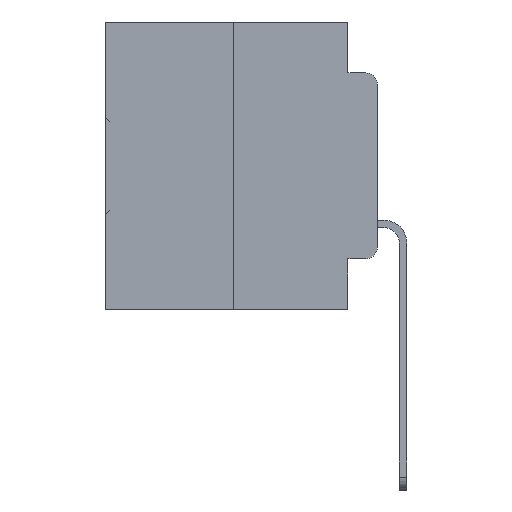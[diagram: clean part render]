
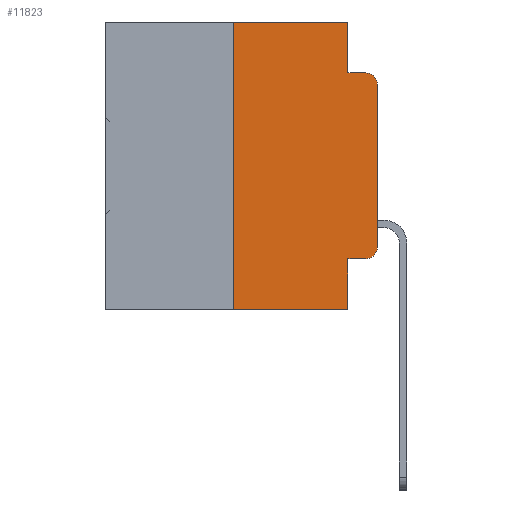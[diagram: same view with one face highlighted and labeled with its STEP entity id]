
A CAD part, left-side view. The second image highlights one B-rep face of the part: STEP entity #11823.
In plain terms, the highlighted planar face has unit normal (-1, 0, 0).
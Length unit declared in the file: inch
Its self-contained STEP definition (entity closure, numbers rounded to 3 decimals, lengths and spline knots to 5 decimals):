
#472 = CIRCLE ( 'NONE', #4220, 0.02 ) ;
#721 = CARTESIAN_POINT ( 'NONE',  ( 0., 0.473, -0.5 ) ) ;
#1151 = VECTOR ( 'NONE', #5588, 39.37008 ) ;
#1259 = ORIENTED_EDGE ( 'NONE', *, *, #29173, .F. ) ;
#1295 = EDGE_CURVE ( 'NONE', #19458, #22076, #29557, .T. ) ;
#1389 = ORIENTED_EDGE ( 'NONE', *, *, #27948, .F. ) ;
#1574 = DIRECTION ( 'NONE',  ( -1., 0., 0. ) ) ;
#1918 = ORIENTED_EDGE ( 'NONE', *, *, #8232, .T. ) ;
#2034 = ORIENTED_EDGE ( 'NONE', *, *, #1295, .T. ) ;
#2562 = LINE ( 'NONE', #23616, #16361 ) ;
#3032 = CARTESIAN_POINT ( 'NONE',  ( 0., 0.02, -0.1085 ) ) ;
#3521 = ORIENTED_EDGE ( 'NONE', *, *, #4174, .F. ) ;
#3566 = ORIENTED_EDGE ( 'NONE', *, *, #13901, .T. ) ;
#3948 = ORIENTED_EDGE ( 'NONE', *, *, #20472, .F. ) ;
#4174 = EDGE_CURVE ( 'NONE', #14409, #23871, #2562, .T. ) ;
#4220 = AXIS2_PLACEMENT_3D ( 'NONE', #18085, #1574, #20760 ) ;
#4297 = DIRECTION ( 'NONE',  ( 0., -1., 0. ) ) ;
#4519 = DIRECTION ( 'NONE',  ( 0., 0., 1. ) ) ;
#4580 = DIRECTION ( 'NONE',  ( 0., 0., -1. ) ) ;
#4784 = ORIENTED_EDGE ( 'NONE', *, *, #31657, .F. ) ;
#4877 = VECTOR ( 'NONE', #19942, 39.37008 ) ;
#5535 = ORIENTED_EDGE ( 'NONE', *, *, #14051, .T. ) ;
#5543 = CARTESIAN_POINT ( 'NONE',  ( 0., 0.051, -0.4115 ) ) ;
#5588 = DIRECTION ( 'NONE',  ( 0., 0., 1. ) ) ;
#5864 = DIRECTION ( 'NONE',  ( 0., 0., -1. ) ) ;
#6602 = DIRECTION ( 'NONE',  ( 0., 0., -1. ) ) ;
#7320 = DIRECTION ( 'NONE',  ( 0., 0., -1. ) ) ;
#8232 = EDGE_CURVE ( 'NONE', #28166, #24749, #30125, .T. ) ;
#8247 = CARTESIAN_POINT ( 'NONE',  ( 0., 0., -0.3915 ) ) ;
#8298 = CARTESIAN_POINT ( 'NONE',  ( 0., 0., -0.1085 ) ) ;
#8684 = CARTESIAN_POINT ( 'NONE',  ( 0., 0.051, 0. ) ) ;
#9003 = ORIENTED_EDGE ( 'NONE', *, *, #16883, .T. ) ;
#9550 = CARTESIAN_POINT ( 'NONE',  ( 0., 0.473, 0. ) ) ;
#11013 = AXIS2_PLACEMENT_3D ( 'NONE', #3032, #22141, #5864 ) ;
#11559 = CIRCLE ( 'NONE', #11013, 0.02 ) ;
#11646 = CARTESIAN_POINT ( 'NONE',  ( 0., 0.051, -0.5 ) ) ;
#11823 = ADVANCED_FACE ( 'NONE', ( #32432 ), #33493, .F. ) ;
#13744 = LINE ( 'NONE', #17960, #28013 ) ;
#13901 = EDGE_CURVE ( 'NONE', #33383, #34877, #26547, .T. ) ;
#14051 = EDGE_CURVE ( 'NONE', #22076, #28166, #472, .T. ) ;
#14409 = VERTEX_POINT ( 'NONE', #8684 ) ;
#15096 = VERTEX_POINT ( 'NONE', #19532 ) ;
#15580 = CARTESIAN_POINT ( 'NONE',  ( 0., 0.25, 0. ) ) ;
#15777 = CARTESIAN_POINT ( 'NONE',  ( 0., 0.051, -0.4115 ) ) ;
#16361 = VECTOR ( 'NONE', #4580, 39.37008 ) ;
#16883 = EDGE_CURVE ( 'NONE', #24749, #22180, #11559, .T. ) ;
#17960 = CARTESIAN_POINT ( 'NONE',  ( 0., 0.051, -0.0885 ) ) ;
#18085 = CARTESIAN_POINT ( 'NONE',  ( 0., 0.02, -0.3915 ) ) ;
#19458 = VERTEX_POINT ( 'NONE', #5543 ) ;
#19532 = CARTESIAN_POINT ( 'NONE',  ( 0., 0.25, 0. ) ) ;
#19942 = DIRECTION ( 'NONE',  ( 0., -1., 0. ) ) ;
#20000 = EDGE_LOOP ( 'NONE', ( #1918, #9003, #4784, #3521, #1389, #1259, #3566, #3948, #2034, #5535 ) ) ;
#20144 = CARTESIAN_POINT ( 'NONE',  ( 0., 0.473, 0. ) ) ;
#20472 = EDGE_CURVE ( 'NONE', #19458, #34877, #27426, .T. ) ;
#20760 = DIRECTION ( 'NONE',  ( 0., 0., -1. ) ) ;
#20811 = CARTESIAN_POINT ( 'NONE',  ( 0., 0.051, -0.0885 ) ) ;
#21526 = CARTESIAN_POINT ( 'NONE',  ( 0., 0.02, -0.0885 ) ) ;
#21879 = CARTESIAN_POINT ( 'NONE',  ( 0., 0., 0. ) ) ;
#22076 = VERTEX_POINT ( 'NONE', #31728 ) ;
#22141 = DIRECTION ( 'NONE',  ( -1., 0., 0. ) ) ;
#22171 = VECTOR ( 'NONE', #4519, 39.37008 ) ;
#22180 = VERTEX_POINT ( 'NONE', #21526 ) ;
#22631 = CARTESIAN_POINT ( 'NONE',  ( 0., 0.25, -0.5 ) ) ;
#22832 = DIRECTION ( 'NONE',  ( 1., 0., 0. ) ) ;
#23616 = CARTESIAN_POINT ( 'NONE',  ( 0., 0.051, 0. ) ) ;
#23871 = VERTEX_POINT ( 'NONE', #20811 ) ;
#24749 = VERTEX_POINT ( 'NONE', #8298 ) ;
#26045 = AXIS2_PLACEMENT_3D ( 'NONE', #20144, #22832, #6602 ) ;
#26547 = LINE ( 'NONE', #721, #4877 ) ;
#27230 = VECTOR ( 'NONE', #28363, 39.37008 ) ;
#27426 = LINE ( 'NONE', #34181, #32895 ) ;
#27861 = VECTOR ( 'NONE', #4297, 39.37008 ) ;
#27948 = EDGE_CURVE ( 'NONE', #15096, #14409, #34359, .T. ) ;
#28013 = VECTOR ( 'NONE', #33994, 39.37008 ) ;
#28166 = VERTEX_POINT ( 'NONE', #8247 ) ;
#28363 = DIRECTION ( 'NONE',  ( 0., -1., 0. ) ) ;
#28415 = LINE ( 'NONE', #15580, #22171 ) ;
#29173 = EDGE_CURVE ( 'NONE', #33383, #15096, #28415, .T. ) ;
#29557 = LINE ( 'NONE', #15777, #27861 ) ;
#30125 = LINE ( 'NONE', #21879, #1151 ) ;
#31657 = EDGE_CURVE ( 'NONE', #23871, #22180, #13744, .T. ) ;
#31728 = CARTESIAN_POINT ( 'NONE',  ( 0., 0.02, -0.4115 ) ) ;
#32432 = FACE_OUTER_BOUND ( 'NONE', #20000, .T. ) ;
#32895 = VECTOR ( 'NONE', #7320, 39.37008 ) ;
#33383 = VERTEX_POINT ( 'NONE', #22631 ) ;
#33493 = PLANE ( 'NONE',  #26045 ) ;
#33994 = DIRECTION ( 'NONE',  ( 0., -1., 0. ) ) ;
#34181 = CARTESIAN_POINT ( 'NONE',  ( 0., 0.051, 0. ) ) ;
#34359 = LINE ( 'NONE', #9550, #27230 ) ;
#34877 = VERTEX_POINT ( 'NONE', #11646 ) ;
